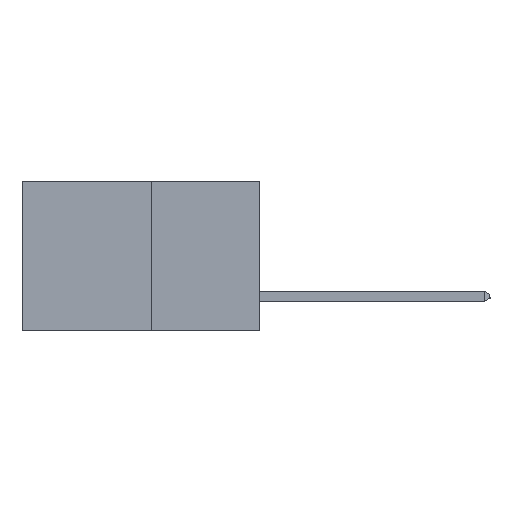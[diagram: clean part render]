
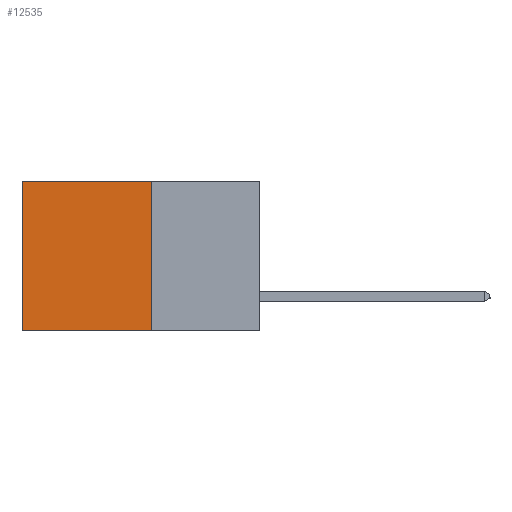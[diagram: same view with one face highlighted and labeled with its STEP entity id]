
A CAD part, left-side view. The second image highlights one B-rep face of the part: STEP entity #12535.
In plain terms, the highlighted planar face has unit normal (-1, 0, 0).
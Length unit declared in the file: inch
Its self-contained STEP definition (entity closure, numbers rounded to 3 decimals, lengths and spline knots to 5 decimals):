
#255 = VERTEX_POINT ( 'NONE', #2350 ) ;
#410 = AXIS2_PLACEMENT_3D ( 'NONE', #8859, #9878, #3700 ) ;
#1184 = VECTOR ( 'NONE', #2598, 39.37008 ) ;
#1447 = LINE ( 'NONE', #9045, #4596 ) ;
#1791 = VERTEX_POINT ( 'NONE', #8470 ) ;
#2350 = CARTESIAN_POINT ( 'NONE',  ( 0.277, 0.27, 0. ) ) ;
#2598 = DIRECTION ( 'NONE',  ( 0., 1., 0. ) ) ;
#2811 = DIRECTION ( 'NONE',  ( 0., 0., -1. ) ) ;
#2911 = FACE_OUTER_BOUND ( 'NONE', #10261, .T. ) ;
#3700 = DIRECTION ( 'NONE',  ( 0., 0., -1. ) ) ;
#4596 = VECTOR ( 'NONE', #2811, 39.37008 ) ;
#5220 = EDGE_CURVE ( 'NONE', #9602, #5483, #8832, .T. ) ;
#5364 = CARTESIAN_POINT ( 'NONE',  ( 0.277, 0.27, -0.37 ) ) ;
#5436 = LINE ( 'NONE', #5364, #13176 ) ;
#5483 = VERTEX_POINT ( 'NONE', #11632 ) ;
#6141 = LINE ( 'NONE', #8844, #1184 ) ;
#6172 = CARTESIAN_POINT ( 'NONE',  ( 0.277, 0.27, -0.37 ) ) ;
#7345 = ORIENTED_EDGE ( 'NONE', *, *, #12015, .T. ) ;
#7814 = PLANE ( 'NONE',  #410 ) ;
#8223 = DIRECTION ( 'NONE',  ( 0., 1., 0. ) ) ;
#8470 = CARTESIAN_POINT ( 'NONE',  ( 0.277, 0.59, 0. ) ) ;
#8832 = LINE ( 'NONE', #6172, #11218 ) ;
#8844 = CARTESIAN_POINT ( 'NONE',  ( 0.277, 0.27, 0. ) ) ;
#8859 = CARTESIAN_POINT ( 'NONE',  ( 0.277, 0.27, -0.37 ) ) ;
#8891 = EDGE_CURVE ( 'NONE', #255, #1791, #6141, .T. ) ;
#9045 = CARTESIAN_POINT ( 'NONE',  ( 0.277, 0.59, -0.37 ) ) ;
#9452 = DIRECTION ( 'NONE',  ( 0., 0., -1. ) ) ;
#9602 = VERTEX_POINT ( 'NONE', #13095 ) ;
#9878 = DIRECTION ( 'NONE',  ( 1., 0., 0. ) ) ;
#10075 = ORIENTED_EDGE ( 'NONE', *, *, #5220, .F. ) ;
#10261 = EDGE_LOOP ( 'NONE', ( #7345, #10075, #12721, #10374 ) ) ;
#10374 = ORIENTED_EDGE ( 'NONE', *, *, #8891, .T. ) ;
#11218 = VECTOR ( 'NONE', #8223, 39.37008 ) ;
#11632 = CARTESIAN_POINT ( 'NONE',  ( 0.277, 0.59, -0.37 ) ) ;
#11718 = EDGE_CURVE ( 'NONE', #255, #9602, #5436, .T. ) ;
#12015 = EDGE_CURVE ( 'NONE', #1791, #5483, #1447, .T. ) ;
#12535 = ADVANCED_FACE ( 'NONE', ( #2911 ), #7814, .F. ) ;
#12721 = ORIENTED_EDGE ( 'NONE', *, *, #11718, .F. ) ;
#13095 = CARTESIAN_POINT ( 'NONE',  ( 0.277, 0.27, -0.37 ) ) ;
#13176 = VECTOR ( 'NONE', #9452, 39.37008 ) ;
